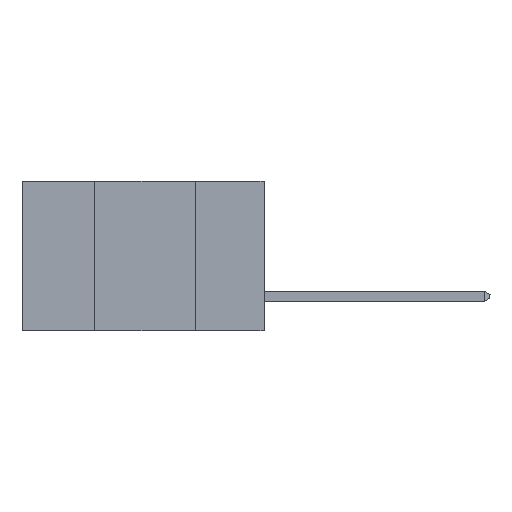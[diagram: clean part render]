
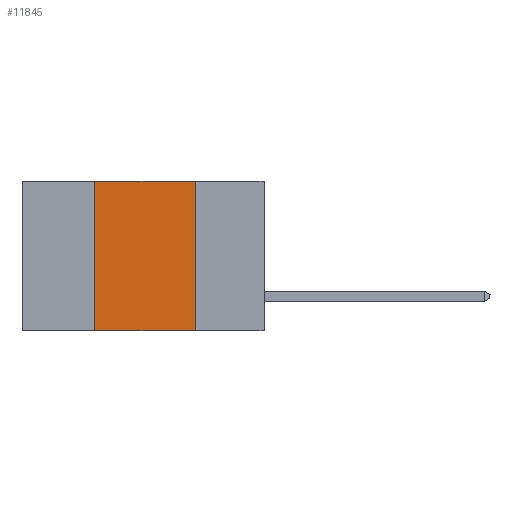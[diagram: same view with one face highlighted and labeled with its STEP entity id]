
A CAD part, left-side view. The second image highlights one B-rep face of the part: STEP entity #11845.
In plain terms, the highlighted planar face has unit normal (-1, 0, 0).
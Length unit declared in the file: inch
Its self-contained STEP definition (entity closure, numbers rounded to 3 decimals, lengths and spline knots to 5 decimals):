
#234 = VECTOR ( 'NONE', #16509, 39.37008 ) ;
#274 = CARTESIAN_POINT ( 'NONE',  ( 0., 0.6, 0. ) ) ;
#753 = ORIENTED_EDGE ( 'NONE', *, *, #13324, .F. ) ;
#2398 = CARTESIAN_POINT ( 'NONE',  ( 0., 0.6, -0.37 ) ) ;
#2717 = CARTESIAN_POINT ( 'NONE',  ( 0., 0.17, 0. ) ) ;
#3459 = VECTOR ( 'NONE', #6187, 39.37008 ) ;
#4685 = EDGE_CURVE ( 'NONE', #11504, #15698, #19494, .T. ) ;
#4897 = VERTEX_POINT ( 'NONE', #2717 ) ;
#5236 = FACE_OUTER_BOUND ( 'NONE', #6605, .T. ) ;
#6187 = DIRECTION ( 'NONE',  ( 0., -1., 0. ) ) ;
#6420 = ORIENTED_EDGE ( 'NONE', *, *, #12702, .T. ) ;
#6605 = EDGE_LOOP ( 'NONE', ( #753, #12439, #19420, #6420 ) ) ;
#7296 = DIRECTION ( 'NONE',  ( 0., 0., -1. ) ) ;
#7979 = EDGE_CURVE ( 'NONE', #15698, #4897, #11783, .T. ) ;
#8998 = VECTOR ( 'NONE', #15463, 39.37008 ) ;
#9627 = CARTESIAN_POINT ( 'NONE',  ( 0., 0.42, -0.37 ) ) ;
#9658 = VERTEX_POINT ( 'NONE', #19617 ) ;
#10648 = DIRECTION ( 'NONE',  ( 1., 0., 0. ) ) ;
#11504 = VERTEX_POINT ( 'NONE', #9627 ) ;
#11585 = CARTESIAN_POINT ( 'NONE',  ( 0., 0.17, -0.37 ) ) ;
#11743 = VECTOR ( 'NONE', #18428, 39.37008 ) ;
#11783 = LINE ( 'NONE', #22087, #11743 ) ;
#11845 = ADVANCED_FACE ( 'NONE', ( #5236 ), #17855, .F. ) ;
#12235 = AXIS2_PLACEMENT_3D ( 'NONE', #274, #10648, #7296 ) ;
#12439 = ORIENTED_EDGE ( 'NONE', *, *, #7979, .F. ) ;
#12702 = EDGE_CURVE ( 'NONE', #11504, #9658, #12856, .T. ) ;
#12856 = LINE ( 'NONE', #2398, #3459 ) ;
#13198 = LINE ( 'NONE', #11585, #8998 ) ;
#13324 = EDGE_CURVE ( 'NONE', #4897, #9658, #13198, .T. ) ;
#15463 = DIRECTION ( 'NONE',  ( 0., 0., -1. ) ) ;
#15698 = VERTEX_POINT ( 'NONE', #20750 ) ;
#16286 = CARTESIAN_POINT ( 'NONE',  ( 0., 0.42, -0.37 ) ) ;
#16509 = DIRECTION ( 'NONE',  ( 0., 0., 1. ) ) ;
#17855 = PLANE ( 'NONE',  #12235 ) ;
#18428 = DIRECTION ( 'NONE',  ( 0., -1., 0. ) ) ;
#19420 = ORIENTED_EDGE ( 'NONE', *, *, #4685, .F. ) ;
#19494 = LINE ( 'NONE', #16286, #234 ) ;
#19617 = CARTESIAN_POINT ( 'NONE',  ( 0., 0.17, -0.37 ) ) ;
#20750 = CARTESIAN_POINT ( 'NONE',  ( 0., 0.42, 0. ) ) ;
#22087 = CARTESIAN_POINT ( 'NONE',  ( 0., 0.6, 0. ) ) ;
